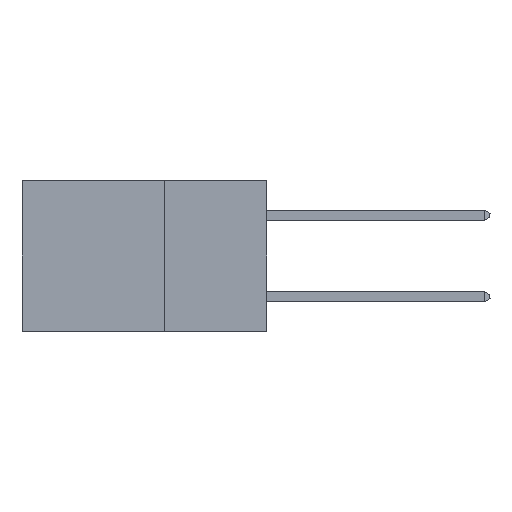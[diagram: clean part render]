
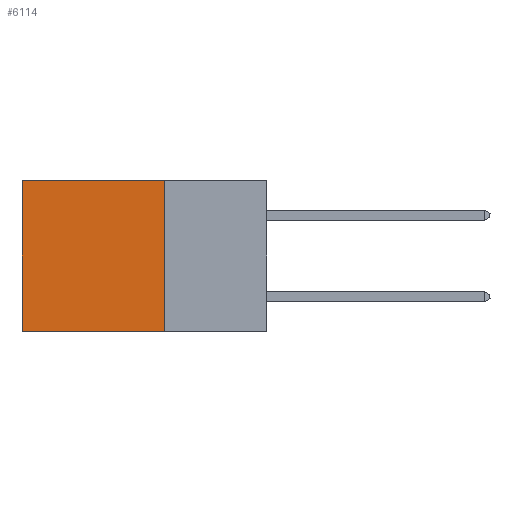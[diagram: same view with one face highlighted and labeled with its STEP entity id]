
A CAD part, left-side view. The second image highlights one B-rep face of the part: STEP entity #6114.
In plain terms, the highlighted planar face has unit normal (-1, 0, 0).
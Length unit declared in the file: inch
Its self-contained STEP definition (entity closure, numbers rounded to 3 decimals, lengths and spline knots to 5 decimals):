
#2506 = LINE ( 'NONE', #40065, #34780 ) ;
#4481 = CARTESIAN_POINT ( 'NONE',  ( 0.2875, 0.25, 0. ) ) ;
#5450 = LINE ( 'NONE', #25805, #29154 ) ;
#6114 = ADVANCED_FACE ( 'NONE', ( #26303 ), #25064, .F. ) ;
#7297 = VERTEX_POINT ( 'NONE', #38250 ) ;
#7513 = EDGE_CURVE ( 'NONE', #43211, #7297, #2506, .T. ) ;
#8393 = DIRECTION ( 'NONE',  ( 0., 1., 0. ) ) ;
#8851 = VECTOR ( 'NONE', #42351, 39.37008 ) ;
#11328 = CARTESIAN_POINT ( 'NONE',  ( 0.2875, 0.25, 0. ) ) ;
#12173 = ORIENTED_EDGE ( 'NONE', *, *, #7513, .T. ) ;
#12715 = EDGE_CURVE ( 'NONE', #31284, #33367, #21762, .T. ) ;
#15433 = AXIS2_PLACEMENT_3D ( 'NONE', #4481, #28374, #24918 ) ;
#21306 = DIRECTION ( 'NONE',  ( 0., 1., 0. ) ) ;
#21762 = LINE ( 'NONE', #38888, #8851 ) ;
#22045 = VECTOR ( 'NONE', #21306, 39.37008 ) ;
#23529 = EDGE_CURVE ( 'NONE', #33367, #7297, #24148, .T. ) ;
#24148 = LINE ( 'NONE', #38464, #22045 ) ;
#24918 = DIRECTION ( 'NONE',  ( 0., 0., -1. ) ) ;
#25064 = PLANE ( 'NONE',  #15433 ) ;
#25220 = CARTESIAN_POINT ( 'NONE',  ( 0.2875, 0.6, 0. ) ) ;
#25805 = CARTESIAN_POINT ( 'NONE',  ( 0.2875, 0.25, 0. ) ) ;
#26303 = FACE_OUTER_BOUND ( 'NONE', #29352, .T. ) ;
#28374 = DIRECTION ( 'NONE',  ( 1., 0., 0. ) ) ;
#29154 = VECTOR ( 'NONE', #8393, 39.37008 ) ;
#29264 = ORIENTED_EDGE ( 'NONE', *, *, #23529, .F. ) ;
#29352 = EDGE_LOOP ( 'NONE', ( #12173, #29264, #43797, #33309 ) ) ;
#29470 = DIRECTION ( 'NONE',  ( 0., 0., -1. ) ) ;
#31284 = VERTEX_POINT ( 'NONE', #11328 ) ;
#33309 = ORIENTED_EDGE ( 'NONE', *, *, #43383, .T. ) ;
#33367 = VERTEX_POINT ( 'NONE', #39322 ) ;
#34780 = VECTOR ( 'NONE', #29470, 39.37008 ) ;
#38250 = CARTESIAN_POINT ( 'NONE',  ( 0.2875, 0.6, -0.37 ) ) ;
#38464 = CARTESIAN_POINT ( 'NONE',  ( 0.2875, 0.25, -0.37 ) ) ;
#38888 = CARTESIAN_POINT ( 'NONE',  ( 0.2875, 0.25, 0. ) ) ;
#39322 = CARTESIAN_POINT ( 'NONE',  ( 0.2875, 0.25, -0.37 ) ) ;
#40065 = CARTESIAN_POINT ( 'NONE',  ( 0.2875, 0.6, 0. ) ) ;
#42351 = DIRECTION ( 'NONE',  ( 0., 0., -1. ) ) ;
#43211 = VERTEX_POINT ( 'NONE', #25220 ) ;
#43383 = EDGE_CURVE ( 'NONE', #31284, #43211, #5450, .T. ) ;
#43797 = ORIENTED_EDGE ( 'NONE', *, *, #12715, .F. ) ;
